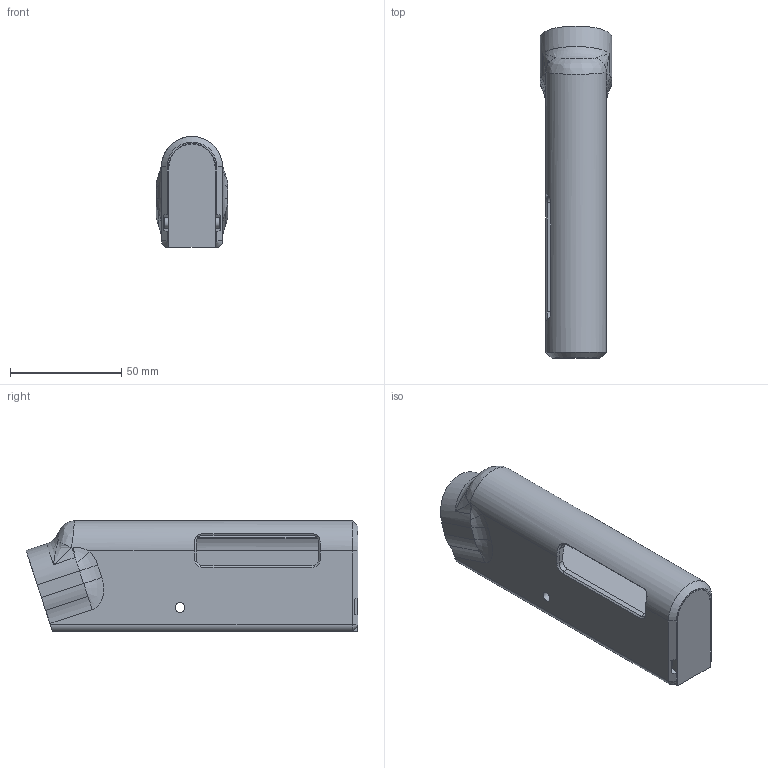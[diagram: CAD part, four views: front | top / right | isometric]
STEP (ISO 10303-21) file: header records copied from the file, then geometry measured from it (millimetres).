
FILE_DESCRIPTION(/* description */ (''),/* implementation_level */ '2;1');
FILE_NAME(/* name */ 'Browning BAR-22 v13.step',/* time_stamp */ '2022-04-09T15:57:21-04:00',/* author */ (''),/* organization */ (''),/* preprocessor_version */ 'ST-DEVELOPER v18.1',/* originating_system */ 'Autodesk Translation Framework v10.14.0.1471',/* authorisation */ '');
FILE_SCHEMA (('AUTOMOTIVE_DESIGN { 1 0 10303 214 3 1 1 }'));
Length unit declared in the file: millimetre
Products named in the file (3): Browning BAR-22; Frame Estimate; Receiver
Assembly tree (2 placements, depth 2):
  Browning BAR-22
    Frame Estimate
    Receiver
Bounding box: 32.32 x 149.21 x 49.9 mm (x, y, z)
Volume: 138442 mm3; surface area: 48653.9 mm2
Topology: 2 solids, 2 shells, 121 faces, 310 edges, 191 vertices
Faces by surface type: plane 59, cylinder 29, bspline 20, cone 8, torus 5
Full cylindrical faces by diameter (mm): 4.35 x1, 4.8 x2, 6 x1, 7.85 x2, 21.6 x1
Entity records: 4517 total; most frequent: CARTESIAN_POINT 1572, ORIENTED_EDGE 612, DIRECTION 570, EDGE_CURVE 306, AXIS2_PLACEMENT_3D 195, VERTEX_POINT 191, LINE 180, VECTOR 180
